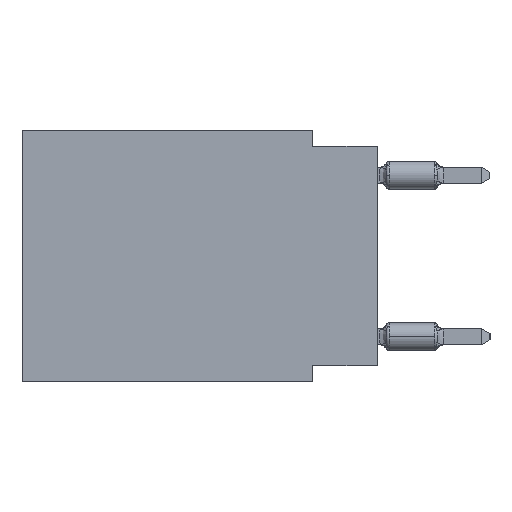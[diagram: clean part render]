
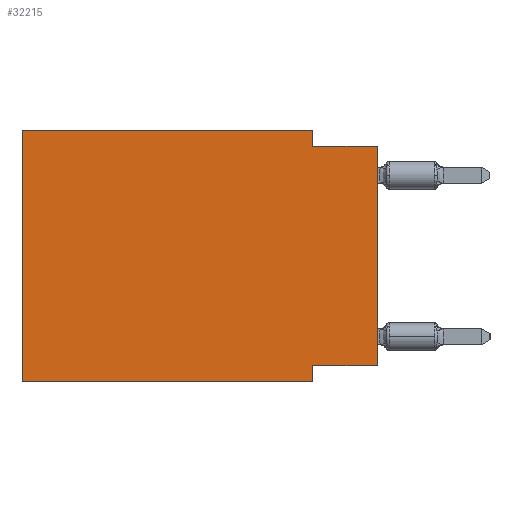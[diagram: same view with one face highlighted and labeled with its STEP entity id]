
A CAD part, left-side view. The second image highlights one B-rep face of the part: STEP entity #32215.
In plain terms, the highlighted planar face has unit normal (-1, 0, 0).
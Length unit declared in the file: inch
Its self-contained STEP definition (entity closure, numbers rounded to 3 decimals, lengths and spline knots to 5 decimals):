
#3099 = CARTESIAN_POINT ( 'NONE',  ( 0., 0., -0.025 ) ) ;
#3280 = EDGE_CURVE ( 'NONE', #7906, #25532, #29354, .T. ) ;
#4709 = PLANE ( 'NONE',  #9289 ) ;
#5542 = CARTESIAN_POINT ( 'NONE',  ( 0., 0.55, -0.39 ) ) ;
#7423 = ORIENTED_EDGE ( 'NONE', *, *, #17125, .F. ) ;
#7906 = VERTEX_POINT ( 'NONE', #31306 ) ;
#9289 = AXIS2_PLACEMENT_3D ( 'NONE', #20872, #33347, #26918 ) ;
#9826 = LINE ( 'NONE', #35132, #15540 ) ;
#11335 = EDGE_CURVE ( 'NONE', #25532, #32724, #9826, .T. ) ;
#11623 = CARTESIAN_POINT ( 'NONE',  ( 0., 0.1, -0.365 ) ) ;
#11703 = CARTESIAN_POINT ( 'NONE',  ( 0., 0.1, -0.025 ) ) ;
#12106 = LINE ( 'NONE', #31436, #30445 ) ;
#12753 = CARTESIAN_POINT ( 'NONE',  ( 0., 0.55, 0. ) ) ;
#13569 = CARTESIAN_POINT ( 'NONE',  ( 0., 0.55, 0. ) ) ;
#14642 = FACE_OUTER_BOUND ( 'NONE', #29207, .T. ) ;
#14963 = CARTESIAN_POINT ( 'NONE',  ( 0., 0.1, 0. ) ) ;
#15540 = VECTOR ( 'NONE', #22276, 39.37008 ) ;
#15735 = EDGE_CURVE ( 'NONE', #38120, #7906, #26033, .T. ) ;
#16028 = VECTOR ( 'NONE', #21916, 39.37008 ) ;
#17125 = EDGE_CURVE ( 'NONE', #35233, #29327, #34415, .T. ) ;
#17615 = CARTESIAN_POINT ( 'NONE',  ( 0., 0., -0.025 ) ) ;
#18108 = CARTESIAN_POINT ( 'NONE',  ( 0., 0.55, -0.39 ) ) ;
#18287 = VERTEX_POINT ( 'NONE', #3099 ) ;
#18519 = ORIENTED_EDGE ( 'NONE', *, *, #3280, .F. ) ;
#19146 = EDGE_CURVE ( 'NONE', #29327, #21950, #12106, .T. ) ;
#19414 = ORIENTED_EDGE ( 'NONE', *, *, #11335, .F. ) ;
#19441 = EDGE_CURVE ( 'NONE', #32724, #18287, #30721, .T. ) ;
#19624 = ORIENTED_EDGE ( 'NONE', *, *, #34812, .T. ) ;
#20872 = CARTESIAN_POINT ( 'NONE',  ( 0., 0.55, 0. ) ) ;
#21225 = ORIENTED_EDGE ( 'NONE', *, *, #19146, .F. ) ;
#21469 = VECTOR ( 'NONE', #31285, 39.37008 ) ;
#21511 = LINE ( 'NONE', #5542, #21469 ) ;
#21916 = DIRECTION ( 'NONE',  ( 0., 0., 1. ) ) ;
#21950 = VERTEX_POINT ( 'NONE', #38351 ) ;
#22276 = DIRECTION ( 'NONE',  ( 0., 0., -1. ) ) ;
#24970 = DIRECTION ( 'NONE',  ( 0., 0., -1. ) ) ;
#25033 = LINE ( 'NONE', #28173, #16028 ) ;
#25532 = VERTEX_POINT ( 'NONE', #14963 ) ;
#26033 = LINE ( 'NONE', #12753, #32347 ) ;
#26346 = EDGE_CURVE ( 'NONE', #38120, #21950, #21511, .T. ) ;
#26844 = DIRECTION ( 'NONE',  ( 0., -1., 0. ) ) ;
#26918 = DIRECTION ( 'NONE',  ( 0., 0., -1. ) ) ;
#27701 = CARTESIAN_POINT ( 'NONE',  ( 0., 0., -0.365 ) ) ;
#28173 = CARTESIAN_POINT ( 'NONE',  ( 0., 0., 0. ) ) ;
#28478 = VECTOR ( 'NONE', #30305, 39.37008 ) ;
#29074 = ORIENTED_EDGE ( 'NONE', *, *, #19441, .F. ) ;
#29115 = ORIENTED_EDGE ( 'NONE', *, *, #15735, .F. ) ;
#29207 = EDGE_LOOP ( 'NONE', ( #19624, #29074, #19414, #18519, #29115, #39938, #21225, #7423 ) ) ;
#29327 = VERTEX_POINT ( 'NONE', #11623 ) ;
#29354 = LINE ( 'NONE', #13569, #29952 ) ;
#29650 = VECTOR ( 'NONE', #38139, 39.37008 ) ;
#29952 = VECTOR ( 'NONE', #26844, 39.37008 ) ;
#30305 = DIRECTION ( 'NONE',  ( 0., -1., 0. ) ) ;
#30445 = VECTOR ( 'NONE', #24970, 39.37008 ) ;
#30721 = LINE ( 'NONE', #17615, #28478 ) ;
#31285 = DIRECTION ( 'NONE',  ( 0., -1., 0. ) ) ;
#31306 = CARTESIAN_POINT ( 'NONE',  ( 0., 0.55, 0. ) ) ;
#31436 = CARTESIAN_POINT ( 'NONE',  ( 0., 0.1, -0.39 ) ) ;
#32215 = ADVANCED_FACE ( 'NONE', ( #14642 ), #4709, .F. ) ;
#32278 = DIRECTION ( 'NONE',  ( 0., 0., 1. ) ) ;
#32347 = VECTOR ( 'NONE', #32278, 39.37008 ) ;
#32724 = VERTEX_POINT ( 'NONE', #11703 ) ;
#33347 = DIRECTION ( 'NONE',  ( 1., 0., 0. ) ) ;
#34415 = LINE ( 'NONE', #37930, #29650 ) ;
#34812 = EDGE_CURVE ( 'NONE', #35233, #18287, #25033, .T. ) ;
#35132 = CARTESIAN_POINT ( 'NONE',  ( 0., 0.1, 0. ) ) ;
#35233 = VERTEX_POINT ( 'NONE', #27701 ) ;
#37930 = CARTESIAN_POINT ( 'NONE',  ( 0., 0., -0.365 ) ) ;
#38120 = VERTEX_POINT ( 'NONE', #18108 ) ;
#38139 = DIRECTION ( 'NONE',  ( 0., 1., 0. ) ) ;
#38351 = CARTESIAN_POINT ( 'NONE',  ( 0., 0.1, -0.39 ) ) ;
#39938 = ORIENTED_EDGE ( 'NONE', *, *, #26346, .T. ) ;
